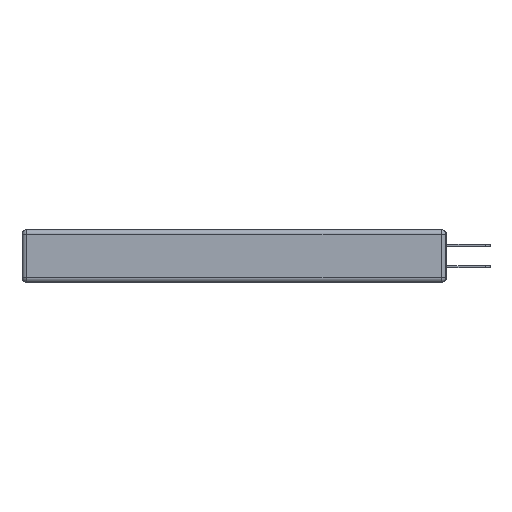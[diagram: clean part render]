
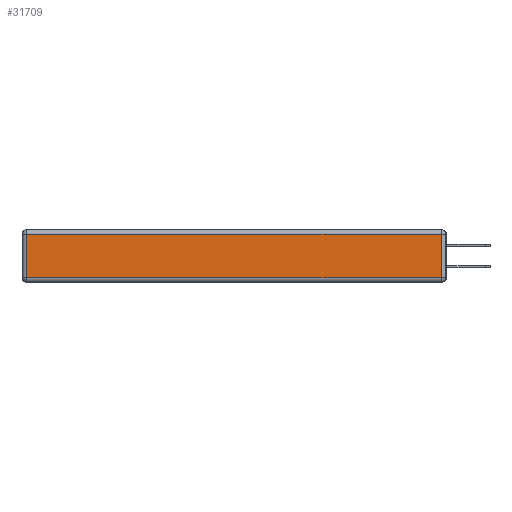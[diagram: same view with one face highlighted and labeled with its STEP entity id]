
A CAD part, left-side view. The second image highlights one B-rep face of the part: STEP entity #31709.
In plain terms, the highlighted planar face has unit normal (-1, 0, 0).
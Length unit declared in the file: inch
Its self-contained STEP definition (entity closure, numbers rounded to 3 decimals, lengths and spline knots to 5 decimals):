
#440 = CARTESIAN_POINT ( 'NONE',  ( 0., 2.72, -0.343 ) ) ;
#1370 = ORIENTED_EDGE ( 'NONE', *, *, #32441, .T. ) ;
#1377 = CARTESIAN_POINT ( 'NONE',  ( 0., 0.03, -0.03 ) ) ;
#1439 = EDGE_CURVE ( 'NONE', #23082, #14158, #3910, .T. ) ;
#1467 = PLANE ( 'NONE',  #9628 ) ;
#3321 = LINE ( 'NONE', #5649, #5679 ) ;
#3910 = LINE ( 'NONE', #25696, #15798 ) ;
#5498 = ORIENTED_EDGE ( 'NONE', *, *, #6652, .T. ) ;
#5521 = ORIENTED_EDGE ( 'NONE', *, *, #27144, .T. ) ;
#5649 = CARTESIAN_POINT ( 'NONE',  ( 0., 0.03, -0.343 ) ) ;
#5679 = VECTOR ( 'NONE', #23199, 39.37008 ) ;
#6652 = EDGE_CURVE ( 'NONE', #14158, #31425, #32844, .T. ) ;
#6703 = EDGE_LOOP ( 'NONE', ( #5521, #1370, #32120, #5498 ) ) ;
#9628 = AXIS2_PLACEMENT_3D ( 'NONE', #11633, #30106, #14519 ) ;
#10725 = CARTESIAN_POINT ( 'NONE',  ( 0., 0., -0.313 ) ) ;
#11633 = CARTESIAN_POINT ( 'NONE',  ( 0., 0., -0.343 ) ) ;
#12769 = VECTOR ( 'NONE', #21189, 39.37008 ) ;
#14116 = CARTESIAN_POINT ( 'NONE',  ( 0., 0.03, -0.313 ) ) ;
#14158 = VERTEX_POINT ( 'NONE', #26539 ) ;
#14519 = DIRECTION ( 'NONE',  ( 0., 0., 1. ) ) ;
#15798 = VECTOR ( 'NONE', #25803, 39.37008 ) ;
#17422 = CARTESIAN_POINT ( 'NONE',  ( 0., 2.72, -0.313 ) ) ;
#18472 = VECTOR ( 'NONE', #20747, 39.37008 ) ;
#20747 = DIRECTION ( 'NONE',  ( 0., 0., -1. ) ) ;
#21189 = DIRECTION ( 'NONE',  ( 0., -1., 0. ) ) ;
#23082 = VERTEX_POINT ( 'NONE', #1377 ) ;
#23174 = VERTEX_POINT ( 'NONE', #14116 ) ;
#23199 = DIRECTION ( 'NONE',  ( 0., 0., 1. ) ) ;
#24640 = LINE ( 'NONE', #10725, #12769 ) ;
#25696 = CARTESIAN_POINT ( 'NONE',  ( 0., 2.75, -0.03 ) ) ;
#25803 = DIRECTION ( 'NONE',  ( 0., 1., 0. ) ) ;
#26012 = FACE_OUTER_BOUND ( 'NONE', #6703, .T. ) ;
#26539 = CARTESIAN_POINT ( 'NONE',  ( 0., 2.72, -0.03 ) ) ;
#27144 = EDGE_CURVE ( 'NONE', #31425, #23174, #24640, .T. ) ;
#30106 = DIRECTION ( 'NONE',  ( -1., 0., 0. ) ) ;
#31425 = VERTEX_POINT ( 'NONE', #17422 ) ;
#31709 = ADVANCED_FACE ( 'NONE', ( #26012 ), #1467, .T. ) ;
#32120 = ORIENTED_EDGE ( 'NONE', *, *, #1439, .T. ) ;
#32441 = EDGE_CURVE ( 'NONE', #23174, #23082, #3321, .T. ) ;
#32844 = LINE ( 'NONE', #440, #18472 ) ;
